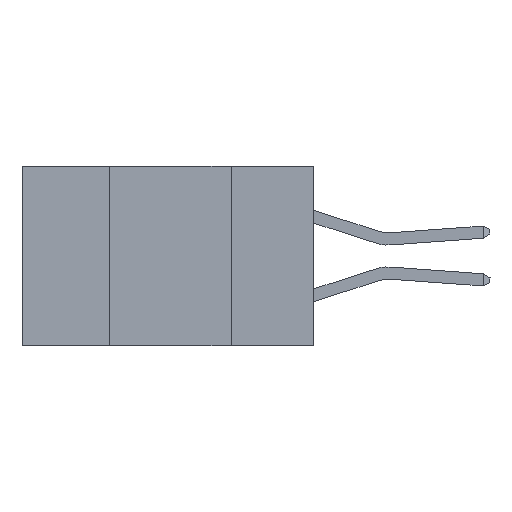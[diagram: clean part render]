
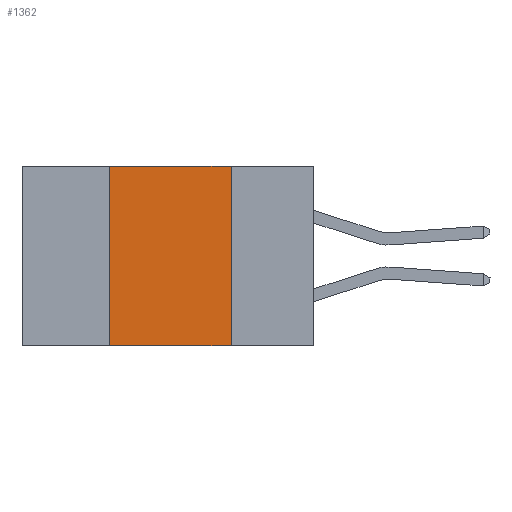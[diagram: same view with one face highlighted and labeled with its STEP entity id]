
A CAD part, left-side view. The second image highlights one B-rep face of the part: STEP entity #1362.
In plain terms, the highlighted planar face has unit normal (-1, 0, 0).
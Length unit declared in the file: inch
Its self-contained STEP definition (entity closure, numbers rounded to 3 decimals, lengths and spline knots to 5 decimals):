
#73 = CARTESIAN_POINT ( 'NONE',  ( 0., 0.42, 0. ) ) ;
#206 = VERTEX_POINT ( 'NONE', #7992 ) ;
#553 = AXIS2_PLACEMENT_3D ( 'NONE', #7940, #4033, #3010 ) ;
#906 = ORIENTED_EDGE ( 'NONE', *, *, #1853, .F. ) ;
#1061 = VERTEX_POINT ( 'NONE', #2080 ) ;
#1302 = CARTESIAN_POINT ( 'NONE',  ( 0., 0.17, 0. ) ) ;
#1362 = ADVANCED_FACE ( 'NONE', ( #11847 ), #4163, .F. ) ;
#1839 = LINE ( 'NONE', #73, #3105 ) ;
#1853 = EDGE_CURVE ( 'NONE', #1061, #4244, #1839, .T. ) ;
#2080 = CARTESIAN_POINT ( 'NONE',  ( 0., 0.42, -0.37 ) ) ;
#2564 = EDGE_CURVE ( 'NONE', #1061, #206, #4618, .T. ) ;
#3010 = DIRECTION ( 'NONE',  ( 0., 0., -1. ) ) ;
#3105 = VECTOR ( 'NONE', #9081, 39.37008 ) ;
#3240 = CARTESIAN_POINT ( 'NONE',  ( 0., 0.6, -0.37 ) ) ;
#3469 = DIRECTION ( 'NONE',  ( 0., 0., -1. ) ) ;
#3707 = VECTOR ( 'NONE', #5334, 39.37008 ) ;
#4033 = DIRECTION ( 'NONE',  ( 1., 0., 0. ) ) ;
#4163 = PLANE ( 'NONE',  #553 ) ;
#4244 = VERTEX_POINT ( 'NONE', #7181 ) ;
#4470 = DIRECTION ( 'NONE',  ( 0., -1., 0. ) ) ;
#4618 = LINE ( 'NONE', #3240, #3707 ) ;
#5334 = DIRECTION ( 'NONE',  ( 0., -1., 0. ) ) ;
#5474 = ORIENTED_EDGE ( 'NONE', *, *, #2564, .T. ) ;
#5795 = EDGE_CURVE ( 'NONE', #4244, #9809, #9005, .T. ) ;
#6024 = ORIENTED_EDGE ( 'NONE', *, *, #5795, .F. ) ;
#6355 = VECTOR ( 'NONE', #4470, 39.37008 ) ;
#6985 = EDGE_LOOP ( 'NONE', ( #11586, #6024, #906, #5474 ) ) ;
#7181 = CARTESIAN_POINT ( 'NONE',  ( 0., 0.42, 0. ) ) ;
#7475 = VECTOR ( 'NONE', #3469, 39.37008 ) ;
#7940 = CARTESIAN_POINT ( 'NONE',  ( 0., 0.6, 0. ) ) ;
#7992 = CARTESIAN_POINT ( 'NONE',  ( 0., 0.17, -0.37 ) ) ;
#9005 = LINE ( 'NONE', #12396, #6355 ) ;
#9081 = DIRECTION ( 'NONE',  ( 0., 0., 1. ) ) ;
#9793 = EDGE_CURVE ( 'NONE', #9809, #206, #11265, .T. ) ;
#9809 = VERTEX_POINT ( 'NONE', #12335 ) ;
#11265 = LINE ( 'NONE', #1302, #7475 ) ;
#11586 = ORIENTED_EDGE ( 'NONE', *, *, #9793, .F. ) ;
#11847 = FACE_OUTER_BOUND ( 'NONE', #6985, .T. ) ;
#12335 = CARTESIAN_POINT ( 'NONE',  ( 0., 0.17, 0. ) ) ;
#12396 = CARTESIAN_POINT ( 'NONE',  ( 0., 0.6, 0. ) ) ;
